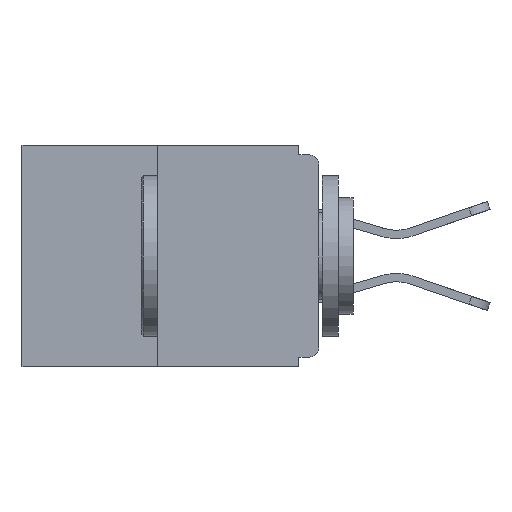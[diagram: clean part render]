
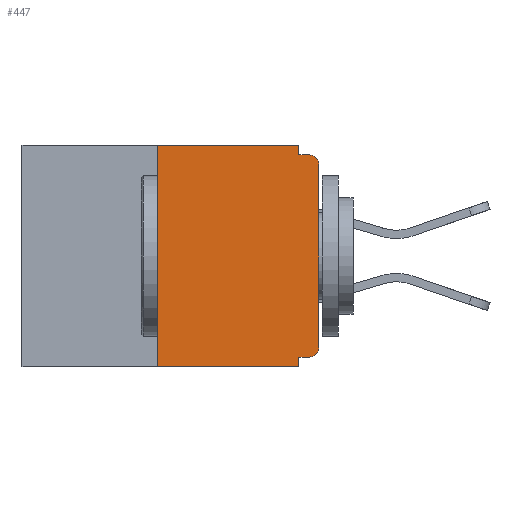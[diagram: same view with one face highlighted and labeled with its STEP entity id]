
A CAD part, left-side view. The second image highlights one B-rep face of the part: STEP entity #447.
In plain terms, the highlighted planar face has unit normal (-1, 0, 0).
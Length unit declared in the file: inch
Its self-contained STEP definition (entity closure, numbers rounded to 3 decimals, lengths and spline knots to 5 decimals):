
#73 = DIRECTION ( 'NONE',  ( 0., 0., 1. ) ) ;
#426 = CARTESIAN_POINT ( 'NONE',  ( 0., 0.031, 0. ) ) ;
#447 = ADVANCED_FACE ( 'NONE', ( #8928 ), #11504, .F. ) ;
#1217 = DIRECTION ( 'NONE',  ( 0., 0., -1. ) ) ;
#1992 = CARTESIAN_POINT ( 'NONE',  ( 0., 0., -0.03 ) ) ;
#2054 = CARTESIAN_POINT ( 'NONE',  ( 0., 0.031, -0.343 ) ) ;
#2115 = LINE ( 'NONE', #2440, #24610 ) ;
#2440 = CARTESIAN_POINT ( 'NONE',  ( 0., 0.25, 0. ) ) ;
#2462 = VERTEX_POINT ( 'NONE', #1992 ) ;
#2507 = LINE ( 'NONE', #13634, #26566 ) ;
#2509 = VERTEX_POINT ( 'NONE', #14560 ) ;
#3045 = LINE ( 'NONE', #3898, #11777 ) ;
#3898 = CARTESIAN_POINT ( 'NONE',  ( 0., 0.46, -0.343 ) ) ;
#4624 = ORIENTED_EDGE ( 'NONE', *, *, #30344, .T. ) ;
#5642 = CARTESIAN_POINT ( 'NONE',  ( 0., 0.031, -0.328 ) ) ;
#5680 = VECTOR ( 'NONE', #19594, 39.37008 ) ;
#6317 = CARTESIAN_POINT ( 'NONE',  ( 0., 0.46, 0. ) ) ;
#6495 = LINE ( 'NONE', #32210, #5680 ) ;
#7122 = CARTESIAN_POINT ( 'NONE',  ( 0., 0., -0.313 ) ) ;
#7270 = VERTEX_POINT ( 'NONE', #21390 ) ;
#7635 = ORIENTED_EDGE ( 'NONE', *, *, #31685, .F. ) ;
#7823 = VERTEX_POINT ( 'NONE', #25036 ) ;
#8544 = DIRECTION ( 'NONE',  ( 0., -1., 0. ) ) ;
#8756 = DIRECTION ( 'NONE',  ( 1., 0., 0. ) ) ;
#8822 = EDGE_LOOP ( 'NONE', ( #11833, #28009, #4624, #16217, #12490, #12712, #27525, #15021, #7635, #12604 ) ) ;
#8884 = EDGE_CURVE ( 'NONE', #15046, #2509, #10896, .T. ) ;
#8895 = AXIS2_PLACEMENT_3D ( 'NONE', #14746, #24876, #24676 ) ;
#8928 = FACE_OUTER_BOUND ( 'NONE', #8822, .T. ) ;
#10206 = LINE ( 'NONE', #2054, #29125 ) ;
#10413 = EDGE_CURVE ( 'NONE', #7823, #18536, #6495, .T. ) ;
#10448 = DIRECTION ( 'NONE',  ( 0., -1., 0. ) ) ;
#10896 = LINE ( 'NONE', #426, #21960 ) ;
#11504 = PLANE ( 'NONE',  #13434 ) ;
#11777 = VECTOR ( 'NONE', #8544, 39.37008 ) ;
#11833 = ORIENTED_EDGE ( 'NONE', *, *, #22583, .F. ) ;
#12490 = ORIENTED_EDGE ( 'NONE', *, *, #10413, .F. ) ;
#12536 = VERTEX_POINT ( 'NONE', #24899 ) ;
#12604 = ORIENTED_EDGE ( 'NONE', *, *, #8884, .F. ) ;
#12712 = ORIENTED_EDGE ( 'NONE', *, *, #17554, .T. ) ;
#13434 = AXIS2_PLACEMENT_3D ( 'NONE', #6317, #8756, #1217 ) ;
#13545 = CARTESIAN_POINT ( 'NONE',  ( 0., 0., -0.015 ) ) ;
#13634 = CARTESIAN_POINT ( 'NONE',  ( 0., 0., 0. ) ) ;
#14196 = CARTESIAN_POINT ( 'NONE',  ( 0., 0.031, 0. ) ) ;
#14560 = CARTESIAN_POINT ( 'NONE',  ( 0., 0.031, -0.015 ) ) ;
#14746 = CARTESIAN_POINT ( 'NONE',  ( 0., 0.015, -0.313 ) ) ;
#15021 = ORIENTED_EDGE ( 'NONE', *, *, #29914, .T. ) ;
#15046 = VERTEX_POINT ( 'NONE', #14196 ) ;
#16217 = ORIENTED_EDGE ( 'NONE', *, *, #24654, .F. ) ;
#17176 = EDGE_CURVE ( 'NONE', #18216, #2462, #2507, .T. ) ;
#17378 = DIRECTION ( 'NONE',  ( 0., 0., -1. ) ) ;
#17554 = EDGE_CURVE ( 'NONE', #7823, #18216, #29326, .T. ) ;
#18216 = VERTEX_POINT ( 'NONE', #7122 ) ;
#18295 = CARTESIAN_POINT ( 'NONE',  ( 0., 0.015, -0.015 ) ) ;
#18536 = VERTEX_POINT ( 'NONE', #5642 ) ;
#18625 = DIRECTION ( 'NONE',  ( 0., -1., 0. ) ) ;
#19594 = DIRECTION ( 'NONE',  ( 0., 1., 0. ) ) ;
#19801 = VECTOR ( 'NONE', #10448, 39.37008 ) ;
#20220 = VERTEX_POINT ( 'NONE', #18295 ) ;
#21071 = CARTESIAN_POINT ( 'NONE',  ( 0., 0.031, -0.343 ) ) ;
#21390 = CARTESIAN_POINT ( 'NONE',  ( 0., 0.25, 0. ) ) ;
#21749 = EDGE_CURVE ( 'NONE', #12536, #7270, #2115, .T. ) ;
#21960 = VECTOR ( 'NONE', #23028, 39.37008 ) ;
#22583 = EDGE_CURVE ( 'NONE', #7270, #15046, #27303, .T. ) ;
#23028 = DIRECTION ( 'NONE',  ( 0., 0., -1. ) ) ;
#23049 = VECTOR ( 'NONE', #18625, 39.37008 ) ;
#24448 = CARTESIAN_POINT ( 'NONE',  ( 0., 0.015, -0.03 ) ) ;
#24610 = VECTOR ( 'NONE', #73, 39.37008 ) ;
#24654 = EDGE_CURVE ( 'NONE', #18536, #26465, #10206, .T. ) ;
#24665 = LINE ( 'NONE', #13545, #23049 ) ;
#24676 = DIRECTION ( 'NONE',  ( 0., 0., -1. ) ) ;
#24876 = DIRECTION ( 'NONE',  ( -1., 0., 0. ) ) ;
#24899 = CARTESIAN_POINT ( 'NONE',  ( 0., 0.25, -0.343 ) ) ;
#25036 = CARTESIAN_POINT ( 'NONE',  ( 0., 0.015, -0.328 ) ) ;
#25738 = CARTESIAN_POINT ( 'NONE',  ( 0., 0.46, 0. ) ) ;
#26465 = VERTEX_POINT ( 'NONE', #21071 ) ;
#26566 = VECTOR ( 'NONE', #31296, 39.37008 ) ;
#27297 = DIRECTION ( 'NONE',  ( 0., 0., -1. ) ) ;
#27303 = LINE ( 'NONE', #25738, #19801 ) ;
#27525 = ORIENTED_EDGE ( 'NONE', *, *, #17176, .T. ) ;
#28009 = ORIENTED_EDGE ( 'NONE', *, *, #21749, .F. ) ;
#29125 = VECTOR ( 'NONE', #27297, 39.37008 ) ;
#29326 = CIRCLE ( 'NONE', #8895, 0.015 ) ;
#29487 = AXIS2_PLACEMENT_3D ( 'NONE', #24448, #32524, #17378 ) ;
#29914 = EDGE_CURVE ( 'NONE', #2462, #20220, #32361, .T. ) ;
#30344 = EDGE_CURVE ( 'NONE', #12536, #26465, #3045, .T. ) ;
#31296 = DIRECTION ( 'NONE',  ( 0., 0., 1. ) ) ;
#31685 = EDGE_CURVE ( 'NONE', #2509, #20220, #24665, .T. ) ;
#32210 = CARTESIAN_POINT ( 'NONE',  ( 0., 0., -0.328 ) ) ;
#32361 = CIRCLE ( 'NONE', #29487, 0.015 ) ;
#32524 = DIRECTION ( 'NONE',  ( -1., 0., 0. ) ) ;
